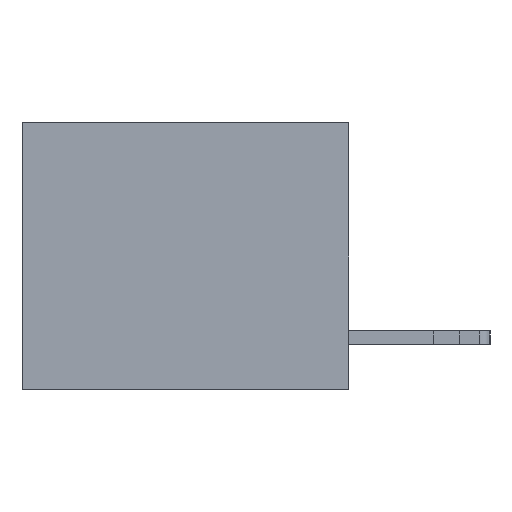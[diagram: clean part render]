
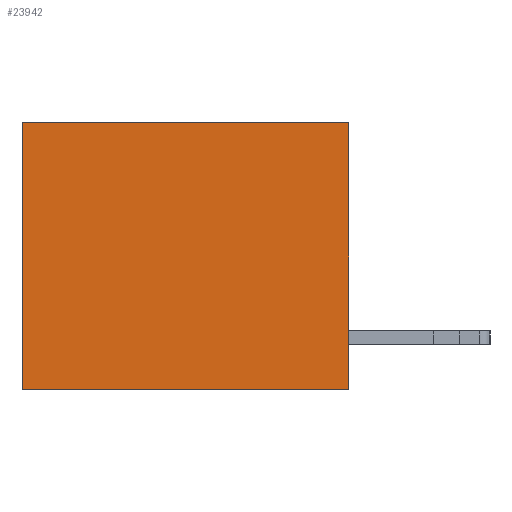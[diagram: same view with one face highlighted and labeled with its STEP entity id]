
A CAD part, left-side view. The second image highlights one B-rep face of the part: STEP entity #23942.
In plain terms, the highlighted planar face has unit normal (-1, 0, 0).
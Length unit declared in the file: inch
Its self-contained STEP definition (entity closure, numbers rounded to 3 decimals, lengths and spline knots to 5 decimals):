
#521 = DIRECTION ( 'NONE',  ( 0., 0., -1. ) ) ;
#581 = ORIENTED_EDGE ( 'NONE', *, *, #15833, .T. ) ;
#2565 = VERTEX_POINT ( 'NONE', #12197 ) ;
#2598 = CARTESIAN_POINT ( 'NONE',  ( 0.3165, 0., 0. ) ) ;
#3569 = CARTESIAN_POINT ( 'NONE',  ( 0.3165, 0., 0. ) ) ;
#3792 = VERTEX_POINT ( 'NONE', #3569 ) ;
#4750 = VECTOR ( 'NONE', #521, 39.37008 ) ;
#6119 = EDGE_LOOP ( 'NONE', ( #581, #6705, #13632, #24144 ) ) ;
#6705 = ORIENTED_EDGE ( 'NONE', *, *, #14469, .F. ) ;
#7027 = CARTESIAN_POINT ( 'NONE',  ( 0.3165, 0.6, -0.49 ) ) ;
#7635 = VECTOR ( 'NONE', #21595, 39.37008 ) ;
#7637 = CARTESIAN_POINT ( 'NONE',  ( 0.3165, 0., -0.49 ) ) ;
#9906 = DIRECTION ( 'NONE',  ( 1., 0., 0. ) ) ;
#9972 = LINE ( 'NONE', #7027, #16739 ) ;
#12197 = CARTESIAN_POINT ( 'NONE',  ( 0.3165, 0., -0.49 ) ) ;
#13632 = ORIENTED_EDGE ( 'NONE', *, *, #16391, .F. ) ;
#13674 = AXIS2_PLACEMENT_3D ( 'NONE', #7637, #9906, #17071 ) ;
#14469 = EDGE_CURVE ( 'NONE', #2565, #29793, #20718, .T. ) ;
#15059 = DIRECTION ( 'NONE',  ( 0., 1., 0. ) ) ;
#15833 = EDGE_CURVE ( 'NONE', #20876, #29793, #9972, .T. ) ;
#16391 = EDGE_CURVE ( 'NONE', #3792, #2565, #17873, .T. ) ;
#16739 = VECTOR ( 'NONE', #23768, 39.37008 ) ;
#16977 = FACE_OUTER_BOUND ( 'NONE', #6119, .T. ) ;
#17071 = DIRECTION ( 'NONE',  ( 0., 0., -1. ) ) ;
#17873 = LINE ( 'NONE', #21798, #4750 ) ;
#17896 = CARTESIAN_POINT ( 'NONE',  ( 0.3165, 0.6, 0. ) ) ;
#18148 = EDGE_CURVE ( 'NONE', #3792, #20876, #23404, .T. ) ;
#19504 = CARTESIAN_POINT ( 'NONE',  ( 0.3165, 0., -0.49 ) ) ;
#20718 = LINE ( 'NONE', #19504, #29357 ) ;
#20876 = VERTEX_POINT ( 'NONE', #17896 ) ;
#21595 = DIRECTION ( 'NONE',  ( 0., 1., 0. ) ) ;
#21798 = CARTESIAN_POINT ( 'NONE',  ( 0.3165, 0., -0.49 ) ) ;
#23404 = LINE ( 'NONE', #2598, #7635 ) ;
#23768 = DIRECTION ( 'NONE',  ( 0., 0., -1. ) ) ;
#23942 = ADVANCED_FACE ( 'NONE', ( #16977 ), #24314, .F. ) ;
#24144 = ORIENTED_EDGE ( 'NONE', *, *, #18148, .T. ) ;
#24314 = PLANE ( 'NONE',  #13674 ) ;
#29357 = VECTOR ( 'NONE', #15059, 39.37008 ) ;
#29686 = CARTESIAN_POINT ( 'NONE',  ( 0.3165, 0.6, -0.49 ) ) ;
#29793 = VERTEX_POINT ( 'NONE', #29686 ) ;
